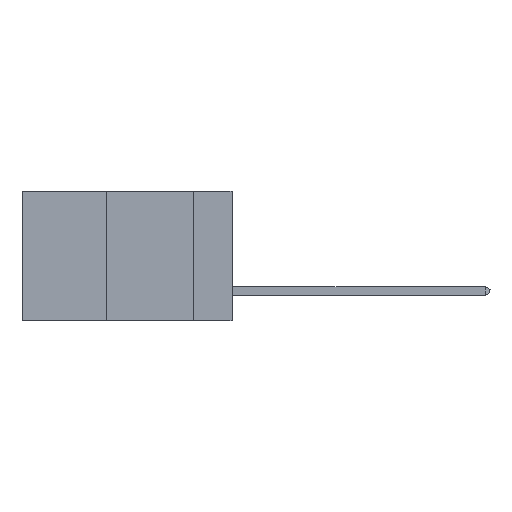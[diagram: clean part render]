
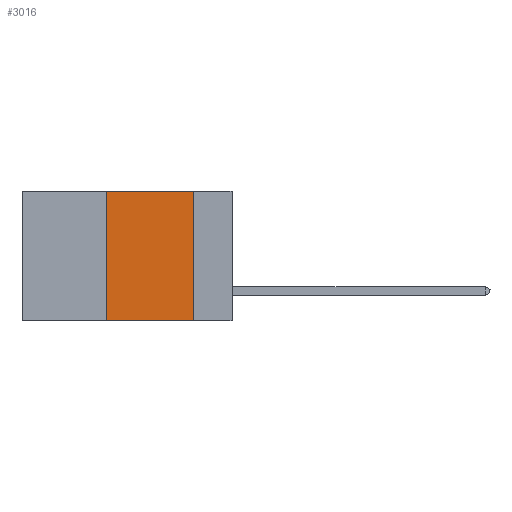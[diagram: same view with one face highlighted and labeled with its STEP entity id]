
A CAD part, left-side view. The second image highlights one B-rep face of the part: STEP entity #3016.
In plain terms, the highlighted planar face has unit normal (-1, 0, 0).
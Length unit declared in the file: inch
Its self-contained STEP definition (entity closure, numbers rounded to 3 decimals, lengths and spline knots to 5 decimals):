
#88 = DIRECTION ( 'NONE',  ( 1., 0., 0. ) ) ;
#589 = EDGE_CURVE ( 'NONE', #1413, #7529, #2068, .T. ) ;
#1413 = VERTEX_POINT ( 'NONE', #8097 ) ;
#2068 = LINE ( 'NONE', #2956, #9656 ) ;
#2903 = EDGE_CURVE ( 'NONE', #10694, #7736, #5821, .T. ) ;
#2956 = CARTESIAN_POINT ( 'NONE',  ( 0., 0.36, 0. ) ) ;
#3016 = ADVANCED_FACE ( 'NONE', ( #5084 ), #10137, .F. ) ;
#3370 = CARTESIAN_POINT ( 'NONE',  ( 0., 0.6, 0. ) ) ;
#3820 = DIRECTION ( 'NONE',  ( 0., -1., 0. ) ) ;
#3854 = EDGE_CURVE ( 'NONE', #7529, #10694, #4146, .T. ) ;
#4146 = LINE ( 'NONE', #3370, #10196 ) ;
#4968 = ORIENTED_EDGE ( 'NONE', *, *, #8761, .T. ) ;
#5084 = FACE_OUTER_BOUND ( 'NONE', #8199, .T. ) ;
#5821 = LINE ( 'NONE', #9257, #10770 ) ;
#6589 = DIRECTION ( 'NONE',  ( 0., 0., -1. ) ) ;
#7529 = VERTEX_POINT ( 'NONE', #10812 ) ;
#7693 = CARTESIAN_POINT ( 'NONE',  ( 0., 0.11, 0. ) ) ;
#7736 = VERTEX_POINT ( 'NONE', #8480 ) ;
#7806 = CARTESIAN_POINT ( 'NONE',  ( 0., 0.6, 0. ) ) ;
#7944 = AXIS2_PLACEMENT_3D ( 'NONE', #7806, #88, #9480 ) ;
#8047 = CARTESIAN_POINT ( 'NONE',  ( 0., 0.6, -0.37 ) ) ;
#8097 = CARTESIAN_POINT ( 'NONE',  ( 0., 0.36, -0.37 ) ) ;
#8199 = EDGE_LOOP ( 'NONE', ( #9276, #9660, #9206, #4968 ) ) ;
#8480 = CARTESIAN_POINT ( 'NONE',  ( 0., 0.11, -0.37 ) ) ;
#8761 = EDGE_CURVE ( 'NONE', #1413, #7736, #10536, .T. ) ;
#9206 = ORIENTED_EDGE ( 'NONE', *, *, #589, .F. ) ;
#9257 = CARTESIAN_POINT ( 'NONE',  ( 0., 0.11, 0. ) ) ;
#9276 = ORIENTED_EDGE ( 'NONE', *, *, #2903, .F. ) ;
#9480 = DIRECTION ( 'NONE',  ( 0., 0., -1. ) ) ;
#9656 = VECTOR ( 'NONE', #9784, 39.37008 ) ;
#9660 = ORIENTED_EDGE ( 'NONE', *, *, #3854, .F. ) ;
#9784 = DIRECTION ( 'NONE',  ( 0., 0., 1. ) ) ;
#9887 = VECTOR ( 'NONE', #3820, 39.37008 ) ;
#10040 = DIRECTION ( 'NONE',  ( 0., -1., 0. ) ) ;
#10137 = PLANE ( 'NONE',  #7944 ) ;
#10196 = VECTOR ( 'NONE', #10040, 39.37008 ) ;
#10536 = LINE ( 'NONE', #8047, #9887 ) ;
#10694 = VERTEX_POINT ( 'NONE', #7693 ) ;
#10770 = VECTOR ( 'NONE', #6589, 39.37008 ) ;
#10812 = CARTESIAN_POINT ( 'NONE',  ( 0., 0.36, 0. ) ) ;
